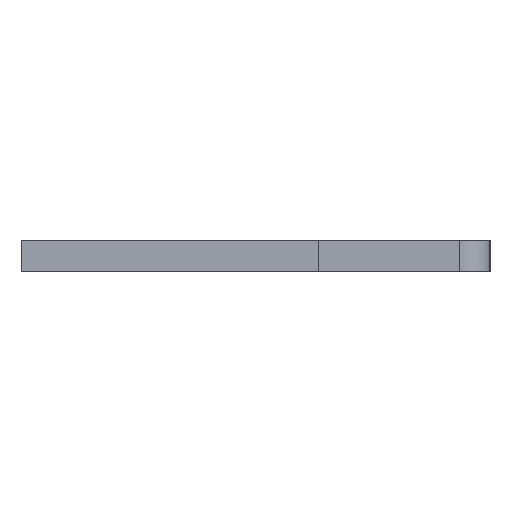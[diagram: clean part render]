
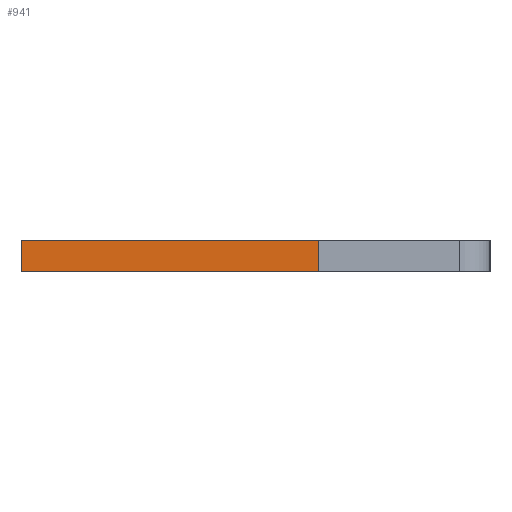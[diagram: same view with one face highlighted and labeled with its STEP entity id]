
A CAD part, left-side view. The second image highlights one B-rep face of the part: STEP entity #941.
In plain terms, the highlighted face is planar.
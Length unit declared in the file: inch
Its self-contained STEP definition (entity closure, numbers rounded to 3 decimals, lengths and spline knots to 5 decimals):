
#3 = VECTOR ( 'NONE', #643, 39.37008 ) ;
#28 = PLANE ( 'NONE',  #543 ) ;
#38 = VERTEX_POINT ( 'NONE', #876 ) ;
#49 = DIRECTION ( 'NONE',  ( -1., 0., 0. ) ) ;
#79 = VERTEX_POINT ( 'NONE', #711 ) ;
#125 = CARTESIAN_POINT ( 'NONE',  ( -0.01, 0.15, -0.04 ) ) ;
#133 = CARTESIAN_POINT ( 'NONE',  ( 0.01, 0.15, -0.04 ) ) ;
#162 = ORIENTED_EDGE ( 'NONE', *, *, #591, .T. ) ;
#223 = EDGE_CURVE ( 'NONE', #448, #38, #517, .T. ) ;
#311 = VERTEX_POINT ( 'NONE', #569 ) ;
#448 = VERTEX_POINT ( 'NONE', #486 ) ;
#467 = DIRECTION ( 'NONE',  ( -1., 0., 0. ) ) ;
#486 = CARTESIAN_POINT ( 'NONE',  ( 0.01, -0.04, -0.04 ) ) ;
#503 = ORIENTED_EDGE ( 'NONE', *, *, #863, .F. ) ;
#506 = DIRECTION ( 'NONE',  ( 1., 0., 0. ) ) ;
#517 = LINE ( 'NONE', #1149, #913 ) ;
#535 = EDGE_CURVE ( 'NONE', #311, #79, #1000, .T. ) ;
#543 = AXIS2_PLACEMENT_3D ( 'NONE', #992, #1088, #506 ) ;
#559 = LINE ( 'NONE', #637, #3 ) ;
#569 = CARTESIAN_POINT ( 'NONE',  ( 0.01, 0.15, -0.04 ) ) ;
#591 = EDGE_CURVE ( 'NONE', #38, #79, #815, .T. ) ;
#595 = DIRECTION ( 'NONE',  ( 0., 1., 0. ) ) ;
#625 = EDGE_LOOP ( 'NONE', ( #162, #1080, #503, #694 ) ) ;
#637 = CARTESIAN_POINT ( 'NONE',  ( 0.01, 0.15, -0.04 ) ) ;
#643 = DIRECTION ( 'NONE',  ( 0., 1., 0. ) ) ;
#694 = ORIENTED_EDGE ( 'NONE', *, *, #223, .T. ) ;
#711 = CARTESIAN_POINT ( 'NONE',  ( -0.01, 0.15, -0.04 ) ) ;
#773 = VECTOR ( 'NONE', #49, 39.37008 ) ;
#815 = LINE ( 'NONE', #125, #923 ) ;
#863 = EDGE_CURVE ( 'NONE', #448, #311, #559, .T. ) ;
#876 = CARTESIAN_POINT ( 'NONE',  ( -0.01, -0.04, -0.04 ) ) ;
#913 = VECTOR ( 'NONE', #467, 39.37008 ) ;
#923 = VECTOR ( 'NONE', #595, 39.37008 ) ;
#941 = ADVANCED_FACE ( 'NONE', ( #982 ), #28, .F. ) ;
#982 = FACE_OUTER_BOUND ( 'NONE', #625, .T. ) ;
#992 = CARTESIAN_POINT ( 'NONE',  ( 0.01, 0.15, -0.04 ) ) ;
#1000 = LINE ( 'NONE', #133, #773 ) ;
#1080 = ORIENTED_EDGE ( 'NONE', *, *, #535, .F. ) ;
#1088 = DIRECTION ( 'NONE',  ( 0., 0., 1. ) ) ;
#1149 = CARTESIAN_POINT ( 'NONE',  ( 0.01, -0.04, -0.04 ) ) ;
